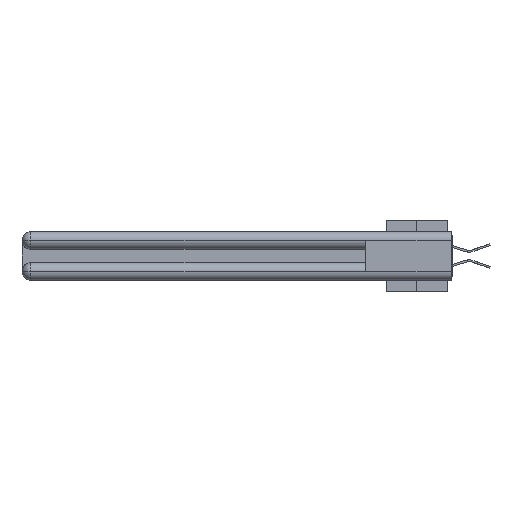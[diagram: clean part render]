
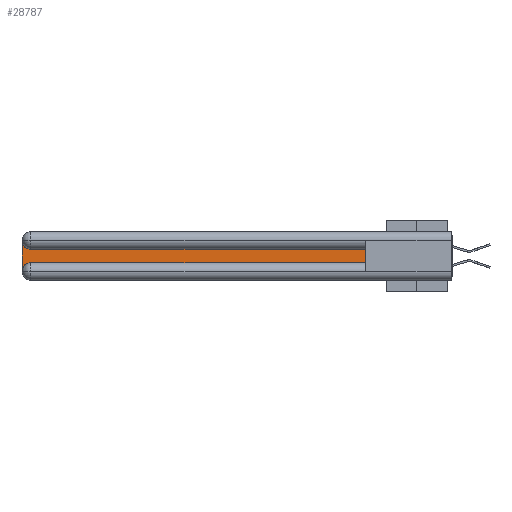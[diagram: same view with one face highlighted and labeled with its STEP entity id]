
A CAD part, left-side view. The second image highlights one B-rep face of the part: STEP entity #28787.
In plain terms, the highlighted planar face has unit normal (-1, 0, 0).
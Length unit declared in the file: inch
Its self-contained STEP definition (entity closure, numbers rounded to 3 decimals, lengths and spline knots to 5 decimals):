
#717 = LINE ( 'NONE', #14530, #1184 ) ;
#1184 = VECTOR ( 'NONE', #5419, 39.37008 ) ;
#2007 = DIRECTION ( 'NONE',  ( 0., 0., 1. ) ) ;
#2235 = EDGE_CURVE ( 'NONE', #8814, #10384, #8962, .T. ) ;
#2965 = VECTOR ( 'NONE', #2007, 39.37008 ) ;
#3264 = CARTESIAN_POINT ( 'NONE',  ( 0.075, 3., -0.0625 ) ) ;
#3692 = CARTESIAN_POINT ( 'NONE',  ( 0.075, 2.94, -0.1225 ) ) ;
#3869 = VERTEX_POINT ( 'NONE', #3692 ) ;
#4617 = ORIENTED_EDGE ( 'NONE', *, *, #5922, .T. ) ;
#5419 = DIRECTION ( 'NONE',  ( 0., 1., 0. ) ) ;
#5916 = CARTESIAN_POINT ( 'NONE',  ( 0.075, 2.94, -0.0625 ) ) ;
#5922 = EDGE_CURVE ( 'NONE', #19087, #8814, #27997, .T. ) ;
#7172 = DIRECTION ( 'NONE',  ( 0., 0., -1. ) ) ;
#7199 = EDGE_CURVE ( 'NONE', #10384, #3869, #717, .T. ) ;
#8048 = ORIENTED_EDGE ( 'NONE', *, *, #7199, .T. ) ;
#8742 = CARTESIAN_POINT ( 'NONE',  ( 0.075, 0.6, -0.2175 ) ) ;
#8771 = VECTOR ( 'NONE', #13794, 39.37008 ) ;
#8814 = VERTEX_POINT ( 'NONE', #8742 ) ;
#8962 = LINE ( 'NONE', #37271, #2965 ) ;
#9232 = DIRECTION ( 'NONE',  ( 0., -1., 0. ) ) ;
#10268 = CARTESIAN_POINT ( 'NONE',  ( 0.075, 3., -0.1225 ) ) ;
#10384 = VERTEX_POINT ( 'NONE', #13752 ) ;
#12715 = CIRCLE ( 'NONE', #36304, 0.06 ) ;
#13752 = CARTESIAN_POINT ( 'NONE',  ( 0.075, 0.6, -0.1225 ) ) ;
#13794 = DIRECTION ( 'NONE',  ( 0., 0., -1. ) ) ;
#14032 = DIRECTION ( 'NONE',  ( 1., 0., 0. ) ) ;
#14530 = CARTESIAN_POINT ( 'NONE',  ( 0.075, 0.6, -0.1225 ) ) ;
#14581 = CIRCLE ( 'NONE', #17209, 0.06 ) ;
#16198 = EDGE_LOOP ( 'NONE', ( #8048, #20955, #22363, #28299, #4617, #17948 ) ) ;
#16387 = PLANE ( 'NONE',  #20965 ) ;
#16745 = CARTESIAN_POINT ( 'NONE',  ( 0.075, 3., -0.2175 ) ) ;
#17209 = AXIS2_PLACEMENT_3D ( 'NONE', #5916, #20434, #26456 ) ;
#17221 = DIRECTION ( 'NONE',  ( 0., 0., -1. ) ) ;
#17948 = ORIENTED_EDGE ( 'NONE', *, *, #2235, .T. ) ;
#19087 = VERTEX_POINT ( 'NONE', #29232 ) ;
#20434 = DIRECTION ( 'NONE',  ( 1., 0., 0. ) ) ;
#20955 = ORIENTED_EDGE ( 'NONE', *, *, #37993, .T. ) ;
#20965 = AXIS2_PLACEMENT_3D ( 'NONE', #10268, #30830, #7172 ) ;
#21210 = LINE ( 'NONE', #16745, #8771 ) ;
#22363 = ORIENTED_EDGE ( 'NONE', *, *, #36444, .T. ) ;
#22773 = CARTESIAN_POINT ( 'NONE',  ( 0.075, 2.94, -0.2775 ) ) ;
#24484 = CARTESIAN_POINT ( 'NONE',  ( 0.075, 3., -0.2775 ) ) ;
#24925 = VERTEX_POINT ( 'NONE', #24484 ) ;
#26456 = DIRECTION ( 'NONE',  ( 0., 0., -1. ) ) ;
#27997 = LINE ( 'NONE', #30312, #34912 ) ;
#28299 = ORIENTED_EDGE ( 'NONE', *, *, #30577, .T. ) ;
#28787 = ADVANCED_FACE ( 'NONE', ( #34438 ), #16387, .F. ) ;
#29232 = CARTESIAN_POINT ( 'NONE',  ( 0.075, 2.94, -0.2175 ) ) ;
#30312 = CARTESIAN_POINT ( 'NONE',  ( 0.075, 0.6, -0.2175 ) ) ;
#30577 = EDGE_CURVE ( 'NONE', #24925, #19087, #12715, .T. ) ;
#30830 = DIRECTION ( 'NONE',  ( 1., 0., 0. ) ) ;
#31947 = VERTEX_POINT ( 'NONE', #3264 ) ;
#34438 = FACE_OUTER_BOUND ( 'NONE', #16198, .T. ) ;
#34912 = VECTOR ( 'NONE', #9232, 39.37008 ) ;
#36304 = AXIS2_PLACEMENT_3D ( 'NONE', #22773, #14032, #17221 ) ;
#36444 = EDGE_CURVE ( 'NONE', #31947, #24925, #21210, .T. ) ;
#37271 = CARTESIAN_POINT ( 'NONE',  ( 0.075, 0.6, -0.2175 ) ) ;
#37993 = EDGE_CURVE ( 'NONE', #3869, #31947, #14581, .T. ) ;
